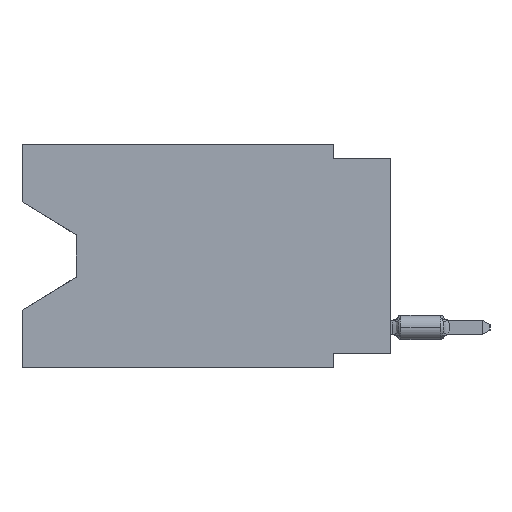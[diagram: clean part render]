
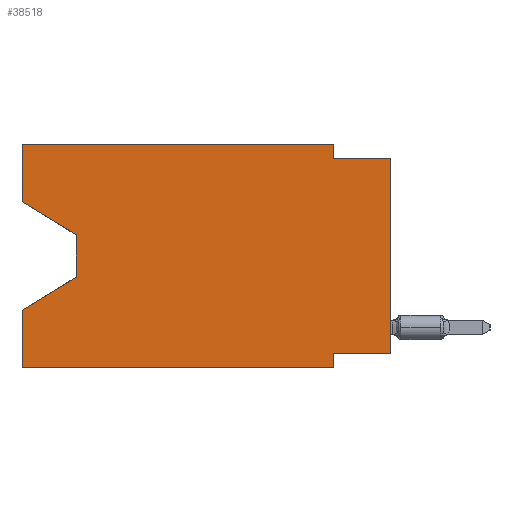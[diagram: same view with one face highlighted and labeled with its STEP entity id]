
A CAD part, left-side view. The second image highlights one B-rep face of the part: STEP entity #38518.
In plain terms, the highlighted planar face has unit normal (-1, 0, 0).
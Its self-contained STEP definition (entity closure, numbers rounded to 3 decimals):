
#248 = DIRECTION ( 'NONE',  ( 0., 1., 0. ) ) ;
#898 = LINE ( 'NONE', #32015, #17138 ) ;
#1608 = DIRECTION ( 'NONE',  ( 0., 0., 1. ) ) ;
#2082 = VECTOR ( 'NONE', #19613, 1000. ) ;
#5412 = LINE ( 'NONE', #42622, #25602 ) ;
#5521 = DIRECTION ( 'NONE',  ( 0., -1., 0. ) ) ;
#6558 = DIRECTION ( 'NONE',  ( 0., -0.855, -0.519 ) ) ;
#6949 = CARTESIAN_POINT ( 'NONE',  ( 0., 0., 0. ) ) ;
#7327 = EDGE_CURVE ( 'NONE', #29323, #31675, #62565, .T. ) ;
#7884 = VERTEX_POINT ( 'NONE', #33414 ) ;
#7980 = ORIENTED_EDGE ( 'NONE', *, *, #51150, .F. ) ;
#8318 = VERTEX_POINT ( 'NONE', #34009 ) ;
#8562 = LINE ( 'NONE', #61518, #66859 ) ;
#8675 = CARTESIAN_POINT ( 'NONE',  ( 0., 16.383, 0. ) ) ;
#9091 = EDGE_LOOP ( 'NONE', ( #64194, #49433, #18649, #62880, #9649, #31988, #52665, #30752, #11560, #7980, #22193, #63440 ) ) ;
#9557 = DIRECTION ( 'NONE',  ( 0., 0., -1. ) ) ;
#9649 = ORIENTED_EDGE ( 'NONE', *, *, #37219, .T. ) ;
#11364 = EDGE_CURVE ( 'NONE', #7884, #31675, #5412, .T. ) ;
#11560 = ORIENTED_EDGE ( 'NONE', *, *, #50189, .F. ) ;
#12368 = CARTESIAN_POINT ( 'NONE',  ( 0., 13.97, -5.893 ) ) ;
#13463 = LINE ( 'NONE', #34640, #52299 ) ;
#13522 = LINE ( 'NONE', #18307, #17674 ) ;
#14836 = LINE ( 'NONE', #66122, #2082 ) ;
#14998 = CARTESIAN_POINT ( 'NONE',  ( 0., 0., -9.271 ) ) ;
#15086 = LINE ( 'NONE', #31489, #56982 ) ;
#15540 = VECTOR ( 'NONE', #30109, 1000. ) ;
#16136 = CARTESIAN_POINT ( 'NONE',  ( 0., 2.54, -9.271 ) ) ;
#17138 = VECTOR ( 'NONE', #67565, 1000. ) ;
#17674 = VECTOR ( 'NONE', #54881, 1000. ) ;
#18307 = CARTESIAN_POINT ( 'NONE',  ( 0., 0., -0.635 ) ) ;
#18649 = ORIENTED_EDGE ( 'NONE', *, *, #7327, .T. ) ;
#19504 = CARTESIAN_POINT ( 'NONE',  ( 0., 2.54, -9.906 ) ) ;
#19613 = DIRECTION ( 'NONE',  ( 0., 0., 1. ) ) ;
#21441 = CARTESIAN_POINT ( 'NONE',  ( 0., 0., -9.271 ) ) ;
#22193 = ORIENTED_EDGE ( 'NONE', *, *, #42660, .F. ) ;
#25602 = VECTOR ( 'NONE', #1608, 1000. ) ;
#25666 = CARTESIAN_POINT ( 'NONE',  ( 0., 2.54, -0.635 ) ) ;
#25687 = EDGE_CURVE ( 'NONE', #65680, #29323, #898, .T. ) ;
#25728 = VECTOR ( 'NONE', #59237, 1000. ) ;
#27601 = VECTOR ( 'NONE', #47847, 1000. ) ;
#28967 = VERTEX_POINT ( 'NONE', #65090 ) ;
#29323 = VERTEX_POINT ( 'NONE', #12368 ) ;
#29348 = EDGE_CURVE ( 'NONE', #8318, #65680, #53386, .T. ) ;
#29531 = DIRECTION ( 'NONE',  ( 1., 0., 0. ) ) ;
#29549 = EDGE_CURVE ( 'NONE', #34048, #44364, #50268, .T. ) ;
#29588 = VERTEX_POINT ( 'NONE', #25666 ) ;
#30109 = DIRECTION ( 'NONE',  ( 0., 0., -1. ) ) ;
#30752 = ORIENTED_EDGE ( 'NONE', *, *, #43843, .T. ) ;
#31489 = CARTESIAN_POINT ( 'NONE',  ( 0., 16.383, 0. ) ) ;
#31675 = VERTEX_POINT ( 'NONE', #36122 ) ;
#31806 = CARTESIAN_POINT ( 'NONE',  ( 0., 13.97, -5.893 ) ) ;
#31988 = ORIENTED_EDGE ( 'NONE', *, *, #29549, .F. ) ;
#32015 = CARTESIAN_POINT ( 'NONE',  ( 0., 13.97, -4.013 ) ) ;
#32255 = LINE ( 'NONE', #6949, #25728 ) ;
#33414 = CARTESIAN_POINT ( 'NONE',  ( 0., 16.383, -9.906 ) ) ;
#34009 = CARTESIAN_POINT ( 'NONE',  ( 0., 16.383, -2.546 ) ) ;
#34048 = VERTEX_POINT ( 'NONE', #16136 ) ;
#34314 = DIRECTION ( 'NONE',  ( 0., -1., 0. ) ) ;
#34640 = CARTESIAN_POINT ( 'NONE',  ( 0., 16.383, -9.906 ) ) ;
#36122 = CARTESIAN_POINT ( 'NONE',  ( 0., 16.383, -7.36 ) ) ;
#37219 = EDGE_CURVE ( 'NONE', #7884, #44364, #13463, .T. ) ;
#37998 = CARTESIAN_POINT ( 'NONE',  ( 0., 16.383, -2.546 ) ) ;
#38518 = ADVANCED_FACE ( 'NONE', ( #44903 ), #65768, .F. ) ;
#41667 = VERTEX_POINT ( 'NONE', #14998 ) ;
#42622 = CARTESIAN_POINT ( 'NONE',  ( 0., 16.383, 0. ) ) ;
#42660 = EDGE_CURVE ( 'NONE', #28967, #55383, #15086, .T. ) ;
#43843 = EDGE_CURVE ( 'NONE', #41667, #46022, #32255, .T. ) ;
#44364 = VERTEX_POINT ( 'NONE', #49792 ) ;
#44903 = FACE_OUTER_BOUND ( 'NONE', #9091, .T. ) ;
#45722 = AXIS2_PLACEMENT_3D ( 'NONE', #8675, #29531, #60953 ) ;
#46022 = VERTEX_POINT ( 'NONE', #64420 ) ;
#46090 = EDGE_CURVE ( 'NONE', #8318, #28967, #14836, .T. ) ;
#46167 = CARTESIAN_POINT ( 'NONE',  ( 0., 2.54, 0. ) ) ;
#46409 = LINE ( 'NONE', #21441, #57679 ) ;
#47847 = DIRECTION ( 'NONE',  ( 0., 0.855, -0.519 ) ) ;
#49433 = ORIENTED_EDGE ( 'NONE', *, *, #25687, .T. ) ;
#49792 = CARTESIAN_POINT ( 'NONE',  ( 0., 2.54, -9.906 ) ) ;
#50189 = EDGE_CURVE ( 'NONE', #29588, #46022, #13522, .T. ) ;
#50268 = LINE ( 'NONE', #19504, #15540 ) ;
#51150 = EDGE_CURVE ( 'NONE', #55383, #29588, #8562, .T. ) ;
#52299 = VECTOR ( 'NONE', #34314, 1000. ) ;
#52665 = ORIENTED_EDGE ( 'NONE', *, *, #66354, .F. ) ;
#53386 = LINE ( 'NONE', #37998, #63484 ) ;
#53721 = CARTESIAN_POINT ( 'NONE',  ( 0., 13.97, -4.013 ) ) ;
#54881 = DIRECTION ( 'NONE',  ( 0., -1., 0. ) ) ;
#55383 = VERTEX_POINT ( 'NONE', #46167 ) ;
#56982 = VECTOR ( 'NONE', #5521, 1000. ) ;
#57679 = VECTOR ( 'NONE', #248, 1000. ) ;
#59237 = DIRECTION ( 'NONE',  ( 0., 0., 1. ) ) ;
#60953 = DIRECTION ( 'NONE',  ( 0., 0., -1. ) ) ;
#61518 = CARTESIAN_POINT ( 'NONE',  ( 0., 2.54, 0. ) ) ;
#62565 = LINE ( 'NONE', #31806, #27601 ) ;
#62880 = ORIENTED_EDGE ( 'NONE', *, *, #11364, .F. ) ;
#63440 = ORIENTED_EDGE ( 'NONE', *, *, #46090, .F. ) ;
#63484 = VECTOR ( 'NONE', #6558, 1000. ) ;
#64194 = ORIENTED_EDGE ( 'NONE', *, *, #29348, .T. ) ;
#64420 = CARTESIAN_POINT ( 'NONE',  ( 0., 0., -0.635 ) ) ;
#65090 = CARTESIAN_POINT ( 'NONE',  ( 0., 16.383, 0. ) ) ;
#65680 = VERTEX_POINT ( 'NONE', #53721 ) ;
#65768 = PLANE ( 'NONE',  #45722 ) ;
#66122 = CARTESIAN_POINT ( 'NONE',  ( 0., 16.383, 0. ) ) ;
#66354 = EDGE_CURVE ( 'NONE', #41667, #34048, #46409, .T. ) ;
#66859 = VECTOR ( 'NONE', #9557, 1000. ) ;
#67565 = DIRECTION ( 'NONE',  ( 0., 0., -1. ) ) ;
